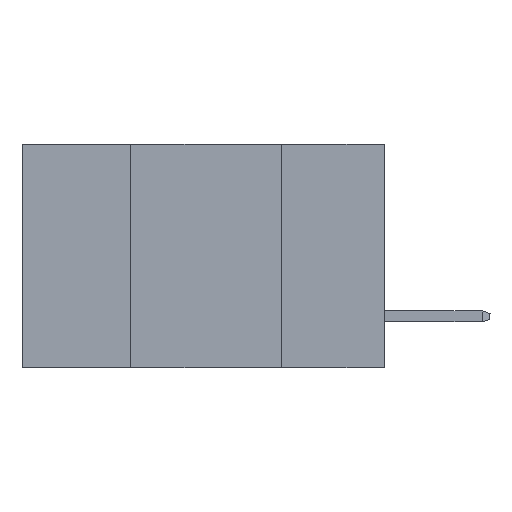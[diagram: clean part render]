
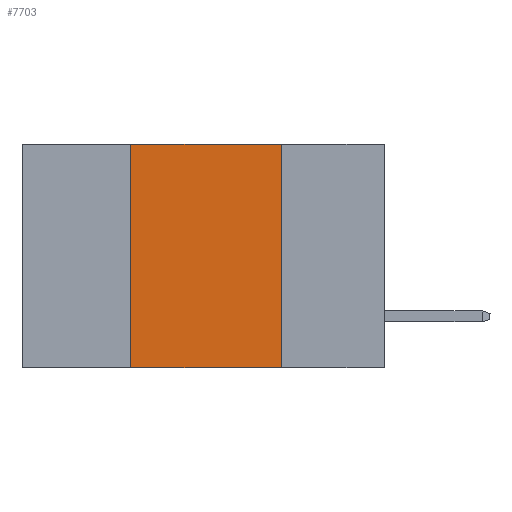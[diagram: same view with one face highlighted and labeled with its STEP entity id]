
A CAD part, left-side view. The second image highlights one B-rep face of the part: STEP entity #7703.
In plain terms, the highlighted planar face has unit normal (-1, 0, 0).
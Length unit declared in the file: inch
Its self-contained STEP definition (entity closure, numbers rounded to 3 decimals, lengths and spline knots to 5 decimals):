
#361 = ORIENTED_EDGE ( 'NONE', *, *, #11040, .F. ) ;
#362 = EDGE_LOOP ( 'NONE', ( #7803, #361, #5151, #3794 ) ) ;
#571 = VERTEX_POINT ( 'NONE', #6084 ) ;
#675 = FACE_OUTER_BOUND ( 'NONE', #362, .T. ) ;
#978 = LINE ( 'NONE', #10020, #13337 ) ;
#1099 = EDGE_CURVE ( 'NONE', #10544, #4743, #978, .T. ) ;
#1543 = LINE ( 'NONE', #13252, #11848 ) ;
#3030 = CARTESIAN_POINT ( 'NONE',  ( 0., 0.6, 0. ) ) ;
#3566 = DIRECTION ( 'NONE',  ( 0., 0., -1. ) ) ;
#3794 = ORIENTED_EDGE ( 'NONE', *, *, #1099, .T. ) ;
#4117 = LINE ( 'NONE', #9906, #14250 ) ;
#4153 = PLANE ( 'NONE',  #7441 ) ;
#4743 = VERTEX_POINT ( 'NONE', #5692 ) ;
#5151 = ORIENTED_EDGE ( 'NONE', *, *, #12757, .F. ) ;
#5391 = DIRECTION ( 'NONE',  ( 0., 0., -1. ) ) ;
#5692 = CARTESIAN_POINT ( 'NONE',  ( 0., 0.17, -0.37 ) ) ;
#6084 = CARTESIAN_POINT ( 'NONE',  ( 0., 0.17, 0. ) ) ;
#7441 = AXIS2_PLACEMENT_3D ( 'NONE', #3030, #12303, #5391 ) ;
#7467 = DIRECTION ( 'NONE',  ( 0., -1., 0. ) ) ;
#7703 = ADVANCED_FACE ( 'NONE', ( #675 ), #4153, .F. ) ;
#7803 = ORIENTED_EDGE ( 'NONE', *, *, #11725, .F. ) ;
#8772 = LINE ( 'NONE', #11036, #9945 ) ;
#9421 = VERTEX_POINT ( 'NONE', #11462 ) ;
#9893 = DIRECTION ( 'NONE',  ( 0., 0., 1. ) ) ;
#9906 = CARTESIAN_POINT ( 'NONE',  ( 0., 0.6, 0. ) ) ;
#9945 = VECTOR ( 'NONE', #9893, 39.37008 ) ;
#10020 = CARTESIAN_POINT ( 'NONE',  ( 0., 0.6, -0.37 ) ) ;
#10544 = VERTEX_POINT ( 'NONE', #11020 ) ;
#11020 = CARTESIAN_POINT ( 'NONE',  ( 0., 0.42, -0.37 ) ) ;
#11036 = CARTESIAN_POINT ( 'NONE',  ( 0., 0.42, -0.37 ) ) ;
#11040 = EDGE_CURVE ( 'NONE', #9421, #571, #4117, .T. ) ;
#11462 = CARTESIAN_POINT ( 'NONE',  ( 0., 0.42, 0. ) ) ;
#11725 = EDGE_CURVE ( 'NONE', #571, #4743, #1543, .T. ) ;
#11848 = VECTOR ( 'NONE', #3566, 39.37008 ) ;
#12303 = DIRECTION ( 'NONE',  ( 1., 0., 0. ) ) ;
#12757 = EDGE_CURVE ( 'NONE', #10544, #9421, #8772, .T. ) ;
#13252 = CARTESIAN_POINT ( 'NONE',  ( 0., 0.17, -0.37 ) ) ;
#13337 = VECTOR ( 'NONE', #14651, 39.37008 ) ;
#14250 = VECTOR ( 'NONE', #7467, 39.37008 ) ;
#14651 = DIRECTION ( 'NONE',  ( 0., -1., 0. ) ) ;
